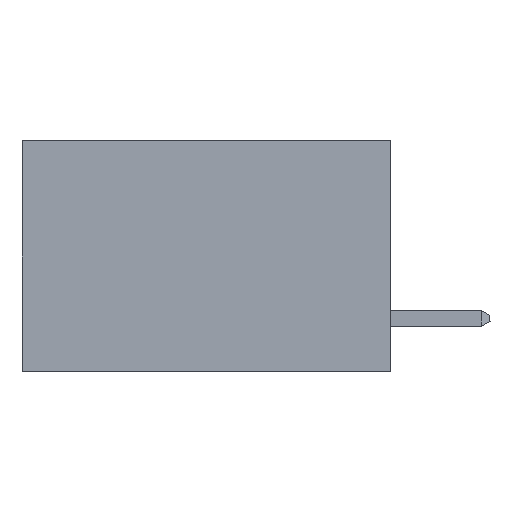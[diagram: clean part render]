
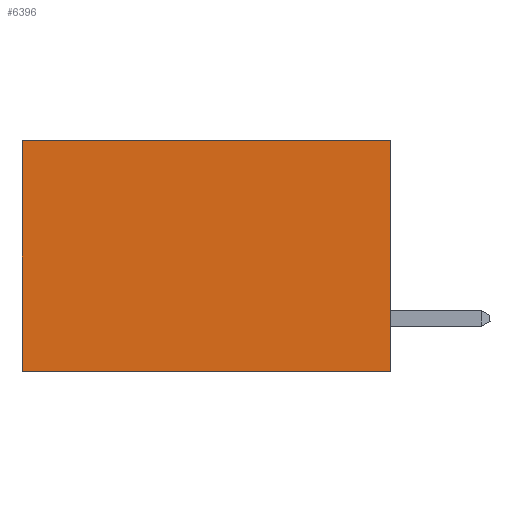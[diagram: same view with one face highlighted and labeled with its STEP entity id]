
A CAD part, left-side view. The second image highlights one B-rep face of the part: STEP entity #6396.
In plain terms, the highlighted planar face has unit normal (-1, 0, 0).
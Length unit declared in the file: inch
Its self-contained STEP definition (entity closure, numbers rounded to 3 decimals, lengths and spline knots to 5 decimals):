
#628 = LINE ( 'NONE', #1858, #6216 ) ;
#777 = VERTEX_POINT ( 'NONE', #11912 ) ;
#1029 = VECTOR ( 'NONE', #4520, 39.37008 ) ;
#1512 = CARTESIAN_POINT ( 'NONE',  ( 0.277, 0.59, 0. ) ) ;
#1570 = VERTEX_POINT ( 'NONE', #1512 ) ;
#1803 = DIRECTION ( 'NONE',  ( 0., 0., -1. ) ) ;
#1858 = CARTESIAN_POINT ( 'NONE',  ( 0.277, 0., -0.37 ) ) ;
#2081 = FACE_OUTER_BOUND ( 'NONE', #10959, .T. ) ;
#2101 = CARTESIAN_POINT ( 'NONE',  ( 0.277, 0., -0.37 ) ) ;
#2290 = CARTESIAN_POINT ( 'NONE',  ( 0.277, 0., -0.37 ) ) ;
#2305 = PLANE ( 'NONE',  #10160 ) ;
#2498 = ORIENTED_EDGE ( 'NONE', *, *, #4759, .T. ) ;
#2581 = ORIENTED_EDGE ( 'NONE', *, *, #6469, .F. ) ;
#2611 = DIRECTION ( 'NONE',  ( 0., 0., -1. ) ) ;
#2613 = ORIENTED_EDGE ( 'NONE', *, *, #10678, .F. ) ;
#2643 = DIRECTION ( 'NONE',  ( 1., 0., 0. ) ) ;
#2954 = ORIENTED_EDGE ( 'NONE', *, *, #12956, .T. ) ;
#3853 = CARTESIAN_POINT ( 'NONE',  ( 0.277, 0., 0. ) ) ;
#4130 = CARTESIAN_POINT ( 'NONE',  ( 0.277, 0.59, -0.37 ) ) ;
#4520 = DIRECTION ( 'NONE',  ( 0., 1., 0. ) ) ;
#4759 = EDGE_CURVE ( 'NONE', #1570, #777, #12443, .T. ) ;
#5304 = VERTEX_POINT ( 'NONE', #11071 ) ;
#5979 = LINE ( 'NONE', #3853, #11193 ) ;
#6216 = VECTOR ( 'NONE', #9478, 39.37008 ) ;
#6396 = ADVANCED_FACE ( 'NONE', ( #2081 ), #2305, .F. ) ;
#6469 = EDGE_CURVE ( 'NONE', #5304, #777, #6956, .T. ) ;
#6942 = VERTEX_POINT ( 'NONE', #10631 ) ;
#6956 = LINE ( 'NONE', #2101, #1029 ) ;
#9158 = DIRECTION ( 'NONE',  ( 0., 1., 0. ) ) ;
#9478 = DIRECTION ( 'NONE',  ( 0., 0., -1. ) ) ;
#9789 = VECTOR ( 'NONE', #1803, 39.37008 ) ;
#10160 = AXIS2_PLACEMENT_3D ( 'NONE', #2290, #2643, #2611 ) ;
#10631 = CARTESIAN_POINT ( 'NONE',  ( 0.277, 0., 0. ) ) ;
#10678 = EDGE_CURVE ( 'NONE', #6942, #5304, #628, .T. ) ;
#10959 = EDGE_LOOP ( 'NONE', ( #2498, #2581, #2613, #2954 ) ) ;
#11071 = CARTESIAN_POINT ( 'NONE',  ( 0.277, 0., -0.37 ) ) ;
#11193 = VECTOR ( 'NONE', #9158, 39.37008 ) ;
#11912 = CARTESIAN_POINT ( 'NONE',  ( 0.277, 0.59, -0.37 ) ) ;
#12443 = LINE ( 'NONE', #4130, #9789 ) ;
#12956 = EDGE_CURVE ( 'NONE', #6942, #1570, #5979, .T. ) ;
